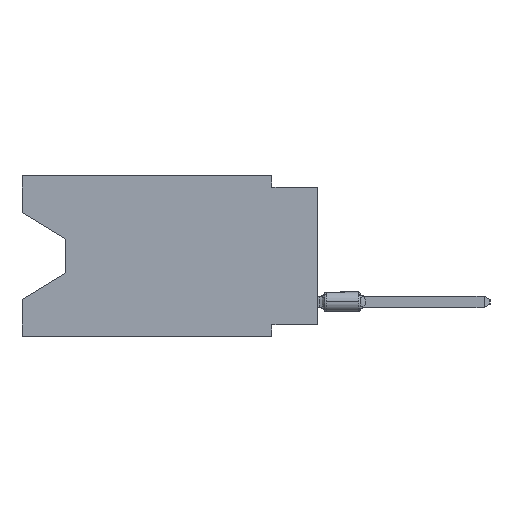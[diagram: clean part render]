
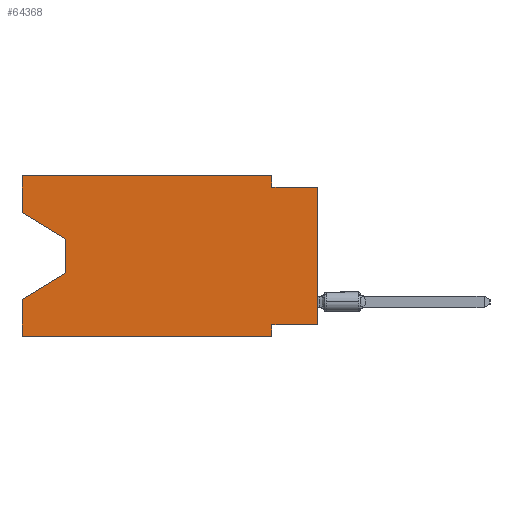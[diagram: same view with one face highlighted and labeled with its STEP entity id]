
A CAD part, left-side view. The second image highlights one B-rep face of the part: STEP entity #64368.
In plain terms, the highlighted planar face has unit normal (-1, 0, 0).
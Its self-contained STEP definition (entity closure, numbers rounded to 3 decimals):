
#1653 = DIRECTION ( 'NONE',  ( 0., 0.855, -0.519 ) ) ;
#1658 = LINE ( 'NONE', #36579, #45587 ) ;
#2099 = VECTOR ( 'NONE', #42189, 1000. ) ;
#2262 = VERTEX_POINT ( 'NONE', #44551 ) ;
#2431 = VECTOR ( 'NONE', #52020, 1000. ) ;
#2672 = ORIENTED_EDGE ( 'NONE', *, *, #44829, .T. ) ;
#2677 = VERTEX_POINT ( 'NONE', #40809 ) ;
#3353 = LINE ( 'NONE', #12170, #2099 ) ;
#5412 = VECTOR ( 'NONE', #34190, 1000. ) ;
#5593 = CARTESIAN_POINT ( 'NONE',  ( 0., 13.97, -3.505 ) ) ;
#7041 = DIRECTION ( 'NONE',  ( 1., 0., 0. ) ) ;
#7329 = VERTEX_POINT ( 'NONE', #52422 ) ;
#9483 = ORIENTED_EDGE ( 'NONE', *, *, #32715, .F. ) ;
#10055 = DIRECTION ( 'NONE',  ( 0., -1., 0. ) ) ;
#10891 = CARTESIAN_POINT ( 'NONE',  ( 0., 2.54, -8.255 ) ) ;
#12170 = CARTESIAN_POINT ( 'NONE',  ( 0., 2.54, 0. ) ) ;
#12195 = VECTOR ( 'NONE', #64273, 1000. ) ;
#13040 = VERTEX_POINT ( 'NONE', #35310 ) ;
#13947 = CARTESIAN_POINT ( 'NONE',  ( 0., 0., 0. ) ) ;
#14204 = DIRECTION ( 'NONE',  ( 0., 0., 1. ) ) ;
#14971 = CARTESIAN_POINT ( 'NONE',  ( 0., 2.54, 0. ) ) ;
#15416 = EDGE_CURVE ( 'NONE', #37345, #13040, #1658, .T. ) ;
#15640 = EDGE_CURVE ( 'NONE', #7329, #52712, #29682, .T. ) ;
#15905 = VERTEX_POINT ( 'NONE', #54342 ) ;
#16522 = PLANE ( 'NONE',  #18796 ) ;
#18130 = VECTOR ( 'NONE', #53116, 1000. ) ;
#18796 = AXIS2_PLACEMENT_3D ( 'NONE', #21729, #7041, #41635 ) ;
#19567 = EDGE_CURVE ( 'NONE', #46409, #63511, #48562, .T. ) ;
#20436 = ORIENTED_EDGE ( 'NONE', *, *, #61637, .F. ) ;
#20825 = EDGE_CURVE ( 'NONE', #15905, #2262, #26464, .T. ) ;
#21264 = DIRECTION ( 'NONE',  ( 0., -1., 0. ) ) ;
#21729 = CARTESIAN_POINT ( 'NONE',  ( 0., 16.383, 0. ) ) ;
#22287 = EDGE_CURVE ( 'NONE', #37345, #2262, #42292, .T. ) ;
#22675 = ORIENTED_EDGE ( 'NONE', *, *, #47492, .T. ) ;
#24074 = CARTESIAN_POINT ( 'NONE',  ( 0., 0., -8.255 ) ) ;
#24589 = ORIENTED_EDGE ( 'NONE', *, *, #33650, .T. ) ;
#26464 = LINE ( 'NONE', #46373, #40636 ) ;
#27165 = CARTESIAN_POINT ( 'NONE',  ( 0., 0., -8.255 ) ) ;
#27207 = VERTEX_POINT ( 'NONE', #14971 ) ;
#27501 = CARTESIAN_POINT ( 'NONE',  ( 0., 16.383, 0. ) ) ;
#27706 = VERTEX_POINT ( 'NONE', #41614 ) ;
#28435 = ORIENTED_EDGE ( 'NONE', *, *, #15640, .F. ) ;
#29637 = CARTESIAN_POINT ( 'NONE',  ( 0., 0., -0.635 ) ) ;
#29682 = LINE ( 'NONE', #34256, #12195 ) ;
#29908 = LINE ( 'NONE', #34485, #50820 ) ;
#31033 = DIRECTION ( 'NONE',  ( 0., 0., -1. ) ) ;
#32016 = ORIENTED_EDGE ( 'NONE', *, *, #58268, .F. ) ;
#32472 = ORIENTED_EDGE ( 'NONE', *, *, #20825, .T. ) ;
#32715 = EDGE_CURVE ( 'NONE', #63511, #13040, #29908, .T. ) ;
#32953 = ORIENTED_EDGE ( 'NONE', *, *, #34744, .F. ) ;
#33090 = CARTESIAN_POINT ( 'NONE',  ( 0., 16.383, -2.038 ) ) ;
#33158 = CARTESIAN_POINT ( 'NONE',  ( 0., 16.383, 0. ) ) ;
#33212 = LINE ( 'NONE', #13947, #18130 ) ;
#33650 = EDGE_CURVE ( 'NONE', #57426, #15905, #40173, .T. ) ;
#34190 = DIRECTION ( 'NONE',  ( 0., 1., 0. ) ) ;
#34256 = CARTESIAN_POINT ( 'NONE',  ( 0., 16.383, 0. ) ) ;
#34485 = CARTESIAN_POINT ( 'NONE',  ( 0., 2.54, -8.89 ) ) ;
#34744 = EDGE_CURVE ( 'NONE', #2677, #27706, #35825, .T. ) ;
#35310 = CARTESIAN_POINT ( 'NONE',  ( 0., 2.54, -8.89 ) ) ;
#35825 = LINE ( 'NONE', #29637, #41559 ) ;
#36579 = CARTESIAN_POINT ( 'NONE',  ( 0., 16.383, -8.89 ) ) ;
#36706 = VECTOR ( 'NONE', #21264, 1000. ) ;
#37345 = VERTEX_POINT ( 'NONE', #39997 ) ;
#39425 = VECTOR ( 'NONE', #31033, 1000. ) ;
#39445 = ORIENTED_EDGE ( 'NONE', *, *, #22287, .F. ) ;
#39863 = ORIENTED_EDGE ( 'NONE', *, *, #15416, .T. ) ;
#39997 = CARTESIAN_POINT ( 'NONE',  ( 0., 16.383, -8.89 ) ) ;
#40173 = LINE ( 'NONE', #5593, #39425 ) ;
#40636 = VECTOR ( 'NONE', #1653, 1000. ) ;
#40809 = CARTESIAN_POINT ( 'NONE',  ( 0., 2.54, -0.635 ) ) ;
#41482 = CARTESIAN_POINT ( 'NONE',  ( 0., 16.383, 0. ) ) ;
#41559 = VECTOR ( 'NONE', #10055, 1000. ) ;
#41614 = CARTESIAN_POINT ( 'NONE',  ( 0., 0., -0.635 ) ) ;
#41635 = DIRECTION ( 'NONE',  ( 0., 0., -1. ) ) ;
#42189 = DIRECTION ( 'NONE',  ( 0., 0., -1. ) ) ;
#42292 = LINE ( 'NONE', #33158, #42875 ) ;
#42875 = VECTOR ( 'NONE', #14204, 1000. ) ;
#44164 = ORIENTED_EDGE ( 'NONE', *, *, #19567, .F. ) ;
#44551 = CARTESIAN_POINT ( 'NONE',  ( 0., 16.383, -6.852 ) ) ;
#44829 = EDGE_CURVE ( 'NONE', #7329, #57426, #52352, .T. ) ;
#45587 = VECTOR ( 'NONE', #61067, 1000. ) ;
#46373 = CARTESIAN_POINT ( 'NONE',  ( 0., 13.97, -5.385 ) ) ;
#46409 = VERTEX_POINT ( 'NONE', #27165 ) ;
#46525 = EDGE_LOOP ( 'NONE', ( #2672, #24589, #32472, #39445, #39863, #9483, #44164, #22675, #32953, #32016, #20436, #28435 ) ) ;
#47492 = EDGE_CURVE ( 'NONE', #46409, #27706, #33212, .T. ) ;
#48562 = LINE ( 'NONE', #24074, #5412 ) ;
#50470 = DIRECTION ( 'NONE',  ( 0., 0., -1. ) ) ;
#50820 = VECTOR ( 'NONE', #50470, 1000. ) ;
#52020 = DIRECTION ( 'NONE',  ( 0., -0.855, -0.519 ) ) ;
#52352 = LINE ( 'NONE', #33090, #2431 ) ;
#52422 = CARTESIAN_POINT ( 'NONE',  ( 0., 16.383, -2.038 ) ) ;
#52712 = VERTEX_POINT ( 'NONE', #27501 ) ;
#53116 = DIRECTION ( 'NONE',  ( 0., 0., 1. ) ) ;
#54342 = CARTESIAN_POINT ( 'NONE',  ( 0., 13.97, -5.385 ) ) ;
#55913 = CARTESIAN_POINT ( 'NONE',  ( 0., 13.97, -3.505 ) ) ;
#56967 = FACE_OUTER_BOUND ( 'NONE', #46525, .T. ) ;
#57426 = VERTEX_POINT ( 'NONE', #55913 ) ;
#58268 = EDGE_CURVE ( 'NONE', #27207, #2677, #3353, .T. ) ;
#61067 = DIRECTION ( 'NONE',  ( 0., -1., 0. ) ) ;
#61637 = EDGE_CURVE ( 'NONE', #52712, #27207, #61717, .T. ) ;
#61717 = LINE ( 'NONE', #41482, #36706 ) ;
#63511 = VERTEX_POINT ( 'NONE', #10891 ) ;
#64273 = DIRECTION ( 'NONE',  ( 0., 0., 1. ) ) ;
#64368 = ADVANCED_FACE ( 'NONE', ( #56967 ), #16522, .F. ) ;
